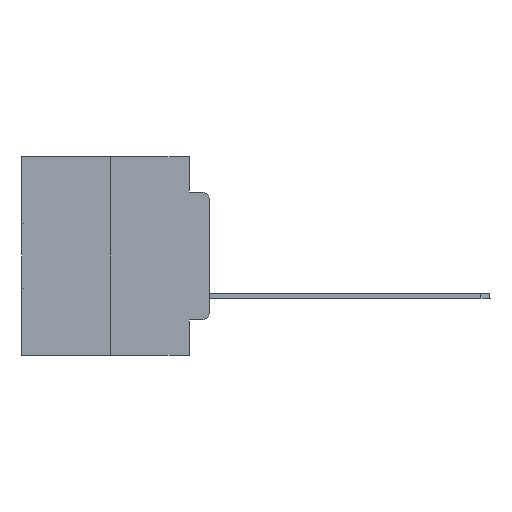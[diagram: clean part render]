
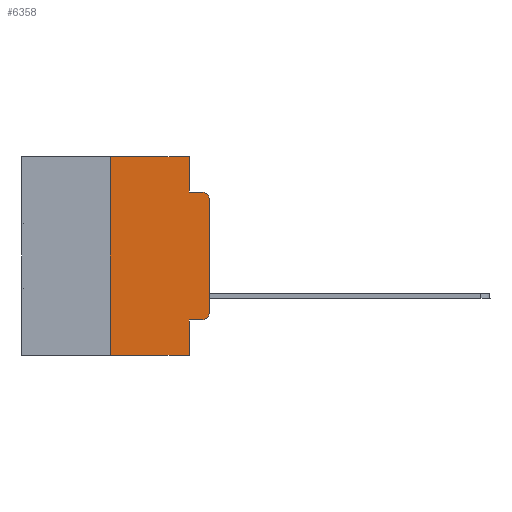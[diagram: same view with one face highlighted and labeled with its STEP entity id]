
A CAD part, left-side view. The second image highlights one B-rep face of the part: STEP entity #6358.
In plain terms, the highlighted planar face has unit normal (-1, 0, 0).
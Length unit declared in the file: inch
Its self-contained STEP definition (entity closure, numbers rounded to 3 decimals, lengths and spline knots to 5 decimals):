
#834 = VECTOR ( 'NONE', #5826, 39.37008 ) ;
#1490 = LINE ( 'NONE', #3702, #18338 ) ;
#1763 = VERTEX_POINT ( 'NONE', #5732 ) ;
#2040 = DIRECTION ( 'NONE',  ( -1., 0., 0. ) ) ;
#2229 = DIRECTION ( 'NONE',  ( 0., 0., -1. ) ) ;
#2719 = LINE ( 'NONE', #8122, #18528 ) ;
#2953 = CARTESIAN_POINT ( 'NONE',  ( 0., 0.25, 0. ) ) ;
#3397 = ORIENTED_EDGE ( 'NONE', *, *, #6416, .T. ) ;
#3602 = DIRECTION ( 'NONE',  ( 0., 0., 1. ) ) ;
#3702 = CARTESIAN_POINT ( 'NONE',  ( 0., 0.25, 0. ) ) ;
#3768 = DIRECTION ( 'NONE',  ( 0., -1., 0. ) ) ;
#3975 = AXIS2_PLACEMENT_3D ( 'NONE', #7294, #5060, #19014 ) ;
#4074 = EDGE_CURVE ( 'NONE', #11003, #24994, #2719, .T. ) ;
#4466 = VERTEX_POINT ( 'NONE', #22611 ) ;
#5060 = DIRECTION ( 'NONE',  ( -1., 0., 0. ) ) ;
#5256 = LINE ( 'NONE', #22910, #22901 ) ;
#5320 = CARTESIAN_POINT ( 'NONE',  ( 0., 0.02, -0.0885 ) ) ;
#5493 = CARTESIAN_POINT ( 'NONE',  ( 0., 0.051, -0.4115 ) ) ;
#5732 = CARTESIAN_POINT ( 'NONE',  ( 0., 0., -0.3915 ) ) ;
#5826 = DIRECTION ( 'NONE',  ( 0., 0., 1. ) ) ;
#6156 = EDGE_CURVE ( 'NONE', #1763, #10414, #16654, .T. ) ;
#6358 = ADVANCED_FACE ( 'NONE', ( #8018 ), #26788, .F. ) ;
#6384 = CARTESIAN_POINT ( 'NONE',  ( 0., 0., 0. ) ) ;
#6416 = EDGE_CURVE ( 'NONE', #4466, #1763, #12337, .T. ) ;
#6465 = CARTESIAN_POINT ( 'NONE',  ( 0., 0.25, -0.5 ) ) ;
#6488 = EDGE_LOOP ( 'NONE', ( #19395, #29175, #19138, #7600, #13030, #12132, #10035, #18480, #25317, #3397 ) ) ;
#7230 = CARTESIAN_POINT ( 'NONE',  ( 0., 0.051, -0.0885 ) ) ;
#7294 = CARTESIAN_POINT ( 'NONE',  ( 0., 0.02, -0.3915 ) ) ;
#7600 = ORIENTED_EDGE ( 'NONE', *, *, #4074, .F. ) ;
#7879 = LINE ( 'NONE', #5493, #13656 ) ;
#8018 = FACE_OUTER_BOUND ( 'NONE', #6488, .T. ) ;
#8067 = CARTESIAN_POINT ( 'NONE',  ( 0., 0.473, 0. ) ) ;
#8122 = CARTESIAN_POINT ( 'NONE',  ( 0., 0.051, 0. ) ) ;
#8901 = CARTESIAN_POINT ( 'NONE',  ( 0., 0.051, -0.0885 ) ) ;
#9268 = CARTESIAN_POINT ( 'NONE',  ( 0., 0.02, -0.1085 ) ) ;
#9934 = DIRECTION ( 'NONE',  ( 0., -1., 0. ) ) ;
#10035 = ORIENTED_EDGE ( 'NONE', *, *, #19003, .T. ) ;
#10414 = VERTEX_POINT ( 'NONE', #26325 ) ;
#10444 = DIRECTION ( 'NONE',  ( 0., 0., -1. ) ) ;
#10681 = CARTESIAN_POINT ( 'NONE',  ( 0., 0.051, -0.5 ) ) ;
#11003 = VERTEX_POINT ( 'NONE', #15498 ) ;
#11007 = LINE ( 'NONE', #7230, #28627 ) ;
#11329 = VERTEX_POINT ( 'NONE', #2953 ) ;
#11437 = EDGE_CURVE ( 'NONE', #11329, #11003, #22337, .T. ) ;
#12079 = EDGE_CURVE ( 'NONE', #10414, #20192, #18637, .T. ) ;
#12132 = ORIENTED_EDGE ( 'NONE', *, *, #27356, .F. ) ;
#12337 = CIRCLE ( 'NONE', #3975, 0.02 ) ;
#13030 = ORIENTED_EDGE ( 'NONE', *, *, #11437, .F. ) ;
#13656 = VECTOR ( 'NONE', #3768, 39.37008 ) ;
#14026 = EDGE_CURVE ( 'NONE', #24994, #20192, #11007, .T. ) ;
#14379 = LINE ( 'NONE', #16699, #15141 ) ;
#15141 = VECTOR ( 'NONE', #16516, 39.37008 ) ;
#15498 = CARTESIAN_POINT ( 'NONE',  ( 0., 0.051, 0. ) ) ;
#15640 = AXIS2_PLACEMENT_3D ( 'NONE', #9268, #2040, #2229 ) ;
#15973 = DIRECTION ( 'NONE',  ( 0., -1., 0. ) ) ;
#16516 = DIRECTION ( 'NONE',  ( 0., 0., -1. ) ) ;
#16644 = VERTEX_POINT ( 'NONE', #6465 ) ;
#16654 = LINE ( 'NONE', #6384, #834 ) ;
#16699 = CARTESIAN_POINT ( 'NONE',  ( 0., 0.051, 0. ) ) ;
#18338 = VECTOR ( 'NONE', #3602, 39.37008 ) ;
#18480 = ORIENTED_EDGE ( 'NONE', *, *, #27815, .F. ) ;
#18528 = VECTOR ( 'NONE', #10444, 39.37008 ) ;
#18637 = CIRCLE ( 'NONE', #15640, 0.02 ) ;
#19003 = EDGE_CURVE ( 'NONE', #16644, #20316, #5256, .T. ) ;
#19014 = DIRECTION ( 'NONE',  ( 0., 0., -1. ) ) ;
#19138 = ORIENTED_EDGE ( 'NONE', *, *, #14026, .F. ) ;
#19395 = ORIENTED_EDGE ( 'NONE', *, *, #6156, .T. ) ;
#19505 = CARTESIAN_POINT ( 'NONE',  ( 0., 0.473, 0. ) ) ;
#20192 = VERTEX_POINT ( 'NONE', #5320 ) ;
#20316 = VERTEX_POINT ( 'NONE', #10681 ) ;
#20759 = VERTEX_POINT ( 'NONE', #27928 ) ;
#21992 = VECTOR ( 'NONE', #26576, 39.37008 ) ;
#22337 = LINE ( 'NONE', #19505, #21992 ) ;
#22477 = AXIS2_PLACEMENT_3D ( 'NONE', #8067, #24159, #28799 ) ;
#22611 = CARTESIAN_POINT ( 'NONE',  ( 0., 0.02, -0.4115 ) ) ;
#22901 = VECTOR ( 'NONE', #15973, 39.37008 ) ;
#22910 = CARTESIAN_POINT ( 'NONE',  ( 0., 0.473, -0.5 ) ) ;
#24159 = DIRECTION ( 'NONE',  ( 1., 0., 0. ) ) ;
#24994 = VERTEX_POINT ( 'NONE', #8901 ) ;
#25317 = ORIENTED_EDGE ( 'NONE', *, *, #28526, .T. ) ;
#26325 = CARTESIAN_POINT ( 'NONE',  ( 0., 0., -0.1085 ) ) ;
#26576 = DIRECTION ( 'NONE',  ( 0., -1., 0. ) ) ;
#26788 = PLANE ( 'NONE',  #22477 ) ;
#27356 = EDGE_CURVE ( 'NONE', #16644, #11329, #1490, .T. ) ;
#27815 = EDGE_CURVE ( 'NONE', #20759, #20316, #14379, .T. ) ;
#27928 = CARTESIAN_POINT ( 'NONE',  ( 0., 0.051, -0.4115 ) ) ;
#28526 = EDGE_CURVE ( 'NONE', #20759, #4466, #7879, .T. ) ;
#28627 = VECTOR ( 'NONE', #9934, 39.37008 ) ;
#28799 = DIRECTION ( 'NONE',  ( 0., 0., -1. ) ) ;
#29175 = ORIENTED_EDGE ( 'NONE', *, *, #12079, .T. ) ;
